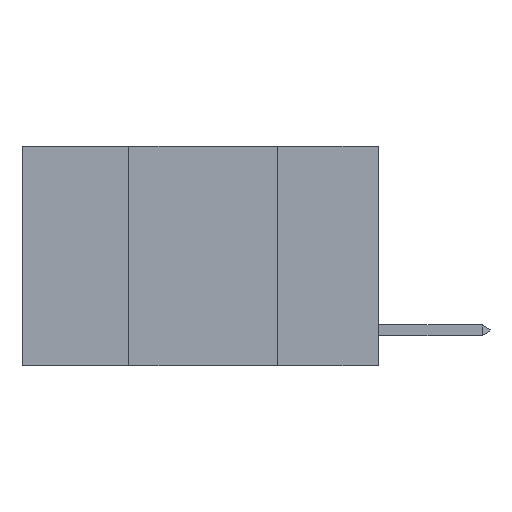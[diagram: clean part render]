
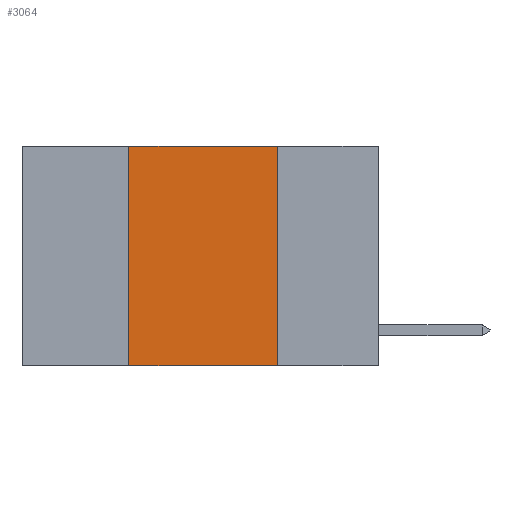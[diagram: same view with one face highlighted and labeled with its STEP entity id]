
A CAD part, left-side view. The second image highlights one B-rep face of the part: STEP entity #3064.
In plain terms, the highlighted planar face has unit normal (-1, 0, 0).
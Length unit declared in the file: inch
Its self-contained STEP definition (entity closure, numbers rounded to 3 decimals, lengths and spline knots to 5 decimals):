
#369 = LINE ( 'NONE', #5700, #11655 ) ;
#395 = ORIENTED_EDGE ( 'NONE', *, *, #11088, .F. ) ;
#744 = VERTEX_POINT ( 'NONE', #3545 ) ;
#1270 = DIRECTION ( 'NONE',  ( 1., 0., 0. ) ) ;
#1961 = VECTOR ( 'NONE', #14128, 39.37008 ) ;
#2590 = VERTEX_POINT ( 'NONE', #6195 ) ;
#2734 = EDGE_LOOP ( 'NONE', ( #8424, #8213, #395, #6349 ) ) ;
#2926 = EDGE_CURVE ( 'NONE', #2590, #3663, #13133, .T. ) ;
#3064 = ADVANCED_FACE ( 'NONE', ( #12289 ), #4616, .F. ) ;
#3545 = CARTESIAN_POINT ( 'NONE',  ( 0., 0.42, 0. ) ) ;
#3604 = DIRECTION ( 'NONE',  ( 0., 0., -1. ) ) ;
#3663 = VERTEX_POINT ( 'NONE', #10787 ) ;
#3963 = VECTOR ( 'NONE', #4184, 39.37008 ) ;
#4184 = DIRECTION ( 'NONE',  ( 0., -1., 0. ) ) ;
#4616 = PLANE ( 'NONE',  #10863 ) ;
#5410 = DIRECTION ( 'NONE',  ( 0., 0., 1. ) ) ;
#5572 = LINE ( 'NONE', #12086, #6098 ) ;
#5648 = CARTESIAN_POINT ( 'NONE',  ( 0., 0.6, 0. ) ) ;
#5700 = CARTESIAN_POINT ( 'NONE',  ( 0., 0.17, 0. ) ) ;
#6098 = VECTOR ( 'NONE', #5410, 39.37008 ) ;
#6144 = CARTESIAN_POINT ( 'NONE',  ( 0., 0.17, 0. ) ) ;
#6195 = CARTESIAN_POINT ( 'NONE',  ( 0., 0.42, -0.37 ) ) ;
#6349 = ORIENTED_EDGE ( 'NONE', *, *, #2926, .T. ) ;
#7117 = EDGE_CURVE ( 'NONE', #11234, #3663, #369, .T. ) ;
#7722 = CARTESIAN_POINT ( 'NONE',  ( 0., 0.6, -0.37 ) ) ;
#7919 = DIRECTION ( 'NONE',  ( 0., 0., -1. ) ) ;
#8213 = ORIENTED_EDGE ( 'NONE', *, *, #14162, .F. ) ;
#8424 = ORIENTED_EDGE ( 'NONE', *, *, #7117, .F. ) ;
#9746 = LINE ( 'NONE', #13062, #3963 ) ;
#10787 = CARTESIAN_POINT ( 'NONE',  ( 0., 0.17, -0.37 ) ) ;
#10863 = AXIS2_PLACEMENT_3D ( 'NONE', #5648, #1270, #3604 ) ;
#11088 = EDGE_CURVE ( 'NONE', #2590, #744, #5572, .T. ) ;
#11234 = VERTEX_POINT ( 'NONE', #6144 ) ;
#11655 = VECTOR ( 'NONE', #7919, 39.37008 ) ;
#12086 = CARTESIAN_POINT ( 'NONE',  ( 0., 0.42, 0. ) ) ;
#12289 = FACE_OUTER_BOUND ( 'NONE', #2734, .T. ) ;
#13062 = CARTESIAN_POINT ( 'NONE',  ( 0., 0.6, 0. ) ) ;
#13133 = LINE ( 'NONE', #7722, #1961 ) ;
#14128 = DIRECTION ( 'NONE',  ( 0., -1., 0. ) ) ;
#14162 = EDGE_CURVE ( 'NONE', #744, #11234, #9746, .T. ) ;
